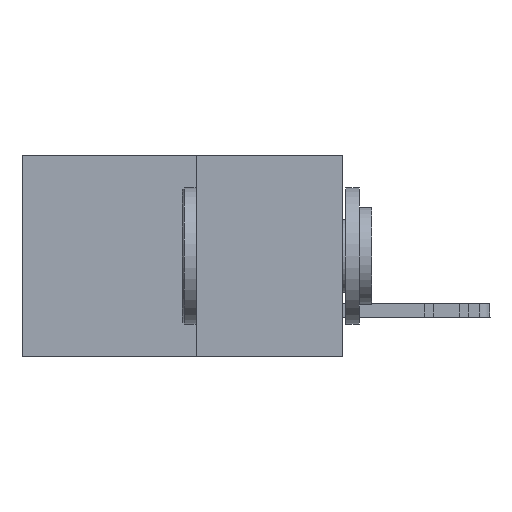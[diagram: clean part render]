
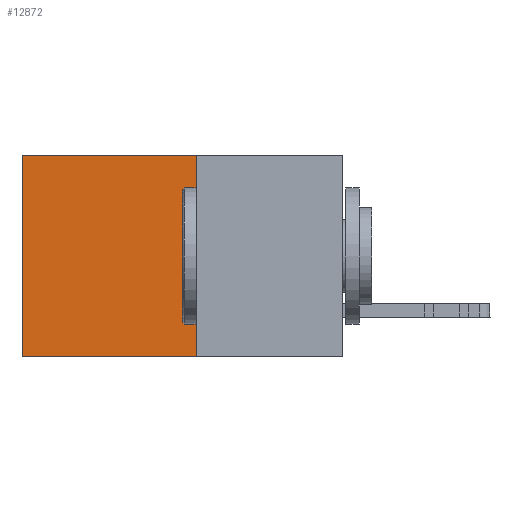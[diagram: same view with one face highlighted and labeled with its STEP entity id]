
A CAD part, left-side view. The second image highlights one B-rep face of the part: STEP entity #12872.
In plain terms, the highlighted planar face has unit normal (-1, 0, 0).
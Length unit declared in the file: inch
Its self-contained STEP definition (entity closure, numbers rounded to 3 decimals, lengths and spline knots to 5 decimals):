
#517 = CARTESIAN_POINT ( 'NONE',  ( 0.277, 0.59, -0.37 ) ) ;
#1608 = CARTESIAN_POINT ( 'NONE',  ( 0.277, 0.27, 0. ) ) ;
#1946 = LINE ( 'NONE', #1608, #22461 ) ;
#3380 = VECTOR ( 'NONE', #10661, 39.37008 ) ;
#3482 = DIRECTION ( 'NONE',  ( 1., 0., 0. ) ) ;
#4532 = VERTEX_POINT ( 'NONE', #13795 ) ;
#4726 = CARTESIAN_POINT ( 'NONE',  ( 0.277, 0.59, -0.37 ) ) ;
#5727 = AXIS2_PLACEMENT_3D ( 'NONE', #16115, #3482, #6130 ) ;
#5922 = CARTESIAN_POINT ( 'NONE',  ( 0.277, 0.27, -0.37 ) ) ;
#6130 = DIRECTION ( 'NONE',  ( 0., 0., -1. ) ) ;
#6209 = LINE ( 'NONE', #23372, #27869 ) ;
#7085 = VERTEX_POINT ( 'NONE', #28262 ) ;
#9839 = EDGE_LOOP ( 'NONE', ( #27326, #22259, #23480, #31301 ) ) ;
#10661 = DIRECTION ( 'NONE',  ( 0., 0., -1. ) ) ;
#11760 = DIRECTION ( 'NONE',  ( 0., 1., 0. ) ) ;
#12872 = ADVANCED_FACE ( 'NONE', ( #23629 ), #30788, .F. ) ;
#13146 = LINE ( 'NONE', #517, #3380 ) ;
#13795 = CARTESIAN_POINT ( 'NONE',  ( 0.277, 0.27, 0. ) ) ;
#14484 = EDGE_CURVE ( 'NONE', #24004, #31923, #21110, .T. ) ;
#16080 = DIRECTION ( 'NONE',  ( 0., 1., 0. ) ) ;
#16115 = CARTESIAN_POINT ( 'NONE',  ( 0.277, 0.27, -0.37 ) ) ;
#18531 = EDGE_CURVE ( 'NONE', #7085, #31923, #13146, .T. ) ;
#19176 = EDGE_CURVE ( 'NONE', #4532, #7085, #1946, .T. ) ;
#21110 = LINE ( 'NONE', #5922, #26411 ) ;
#21361 = EDGE_CURVE ( 'NONE', #4532, #24004, #6209, .T. ) ;
#21707 = CARTESIAN_POINT ( 'NONE',  ( 0.277, 0.27, -0.37 ) ) ;
#22259 = ORIENTED_EDGE ( 'NONE', *, *, #14484, .F. ) ;
#22461 = VECTOR ( 'NONE', #11760, 39.37008 ) ;
#23372 = CARTESIAN_POINT ( 'NONE',  ( 0.277, 0.27, -0.37 ) ) ;
#23480 = ORIENTED_EDGE ( 'NONE', *, *, #21361, .F. ) ;
#23629 = FACE_OUTER_BOUND ( 'NONE', #9839, .T. ) ;
#24004 = VERTEX_POINT ( 'NONE', #21707 ) ;
#26411 = VECTOR ( 'NONE', #16080, 39.37008 ) ;
#27326 = ORIENTED_EDGE ( 'NONE', *, *, #18531, .T. ) ;
#27869 = VECTOR ( 'NONE', #28361, 39.37008 ) ;
#28262 = CARTESIAN_POINT ( 'NONE',  ( 0.277, 0.59, 0. ) ) ;
#28361 = DIRECTION ( 'NONE',  ( 0., 0., -1. ) ) ;
#30788 = PLANE ( 'NONE',  #5727 ) ;
#31301 = ORIENTED_EDGE ( 'NONE', *, *, #19176, .T. ) ;
#31923 = VERTEX_POINT ( 'NONE', #4726 ) ;
